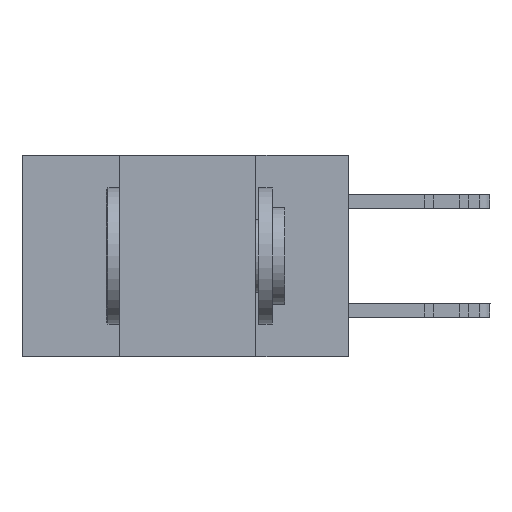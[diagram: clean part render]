
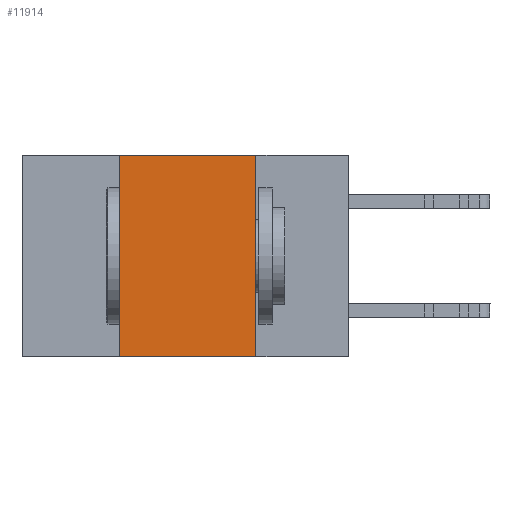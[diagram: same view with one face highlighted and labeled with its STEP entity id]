
A CAD part, left-side view. The second image highlights one B-rep face of the part: STEP entity #11914.
In plain terms, the highlighted planar face has unit normal (-1, 0, 0).
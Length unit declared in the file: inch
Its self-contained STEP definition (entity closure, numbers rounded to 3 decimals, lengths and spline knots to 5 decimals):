
#1058 = FACE_OUTER_BOUND ( 'NONE', #21331, .T. ) ;
#1411 = ORIENTED_EDGE ( 'NONE', *, *, #20245, .F. ) ;
#2018 = ORIENTED_EDGE ( 'NONE', *, *, #11762, .F. ) ;
#2824 = VECTOR ( 'NONE', #12751, 39.37008 ) ;
#3427 = VECTOR ( 'NONE', #4857, 39.37008 ) ;
#3607 = VERTEX_POINT ( 'NONE', #22484 ) ;
#3925 = CARTESIAN_POINT ( 'NONE',  ( 0., 0.6, 0. ) ) ;
#4857 = DIRECTION ( 'NONE',  ( 0., 0., 1. ) ) ;
#5478 = CARTESIAN_POINT ( 'NONE',  ( 0., 0.42, -0.37 ) ) ;
#5915 = DIRECTION ( 'NONE',  ( 0., 0., -1. ) ) ;
#6021 = AXIS2_PLACEMENT_3D ( 'NONE', #3925, #17808, #5915 ) ;
#6224 = VERTEX_POINT ( 'NONE', #18409 ) ;
#8530 = ORIENTED_EDGE ( 'NONE', *, *, #17614, .F. ) ;
#8758 = CARTESIAN_POINT ( 'NONE',  ( 0., 0.6, -0.37 ) ) ;
#9326 = LINE ( 'NONE', #12823, #3427 ) ;
#10775 = VECTOR ( 'NONE', #17611, 39.37008 ) ;
#11757 = VERTEX_POINT ( 'NONE', #5478 ) ;
#11762 = EDGE_CURVE ( 'NONE', #23417, #6224, #19010, .T. ) ;
#11914 = ADVANCED_FACE ( 'NONE', ( #1058 ), #15811, .F. ) ;
#12751 = DIRECTION ( 'NONE',  ( 0., -1., 0. ) ) ;
#12823 = CARTESIAN_POINT ( 'NONE',  ( 0., 0.42, -0.37 ) ) ;
#13323 = CARTESIAN_POINT ( 'NONE',  ( 0., 0.42, 0. ) ) ;
#13375 = LINE ( 'NONE', #8758, #2824 ) ;
#13595 = EDGE_CURVE ( 'NONE', #11757, #3607, #13375, .T. ) ;
#14423 = ORIENTED_EDGE ( 'NONE', *, *, #13595, .T. ) ;
#15811 = PLANE ( 'NONE',  #6021 ) ;
#16055 = LINE ( 'NONE', #19584, #10775 ) ;
#17387 = CARTESIAN_POINT ( 'NONE',  ( 0., 0.6, 0. ) ) ;
#17611 = DIRECTION ( 'NONE',  ( 0., 0., -1. ) ) ;
#17614 = EDGE_CURVE ( 'NONE', #11757, #23417, #9326, .T. ) ;
#17808 = DIRECTION ( 'NONE',  ( 1., 0., 0. ) ) ;
#18409 = CARTESIAN_POINT ( 'NONE',  ( 0., 0.17, 0. ) ) ;
#19010 = LINE ( 'NONE', #17387, #23647 ) ;
#19584 = CARTESIAN_POINT ( 'NONE',  ( 0., 0.17, -0.37 ) ) ;
#20245 = EDGE_CURVE ( 'NONE', #6224, #3607, #16055, .T. ) ;
#21331 = EDGE_LOOP ( 'NONE', ( #1411, #2018, #8530, #14423 ) ) ;
#21364 = DIRECTION ( 'NONE',  ( 0., -1., 0. ) ) ;
#22484 = CARTESIAN_POINT ( 'NONE',  ( 0., 0.17, -0.37 ) ) ;
#23417 = VERTEX_POINT ( 'NONE', #13323 ) ;
#23647 = VECTOR ( 'NONE', #21364, 39.37008 ) ;
